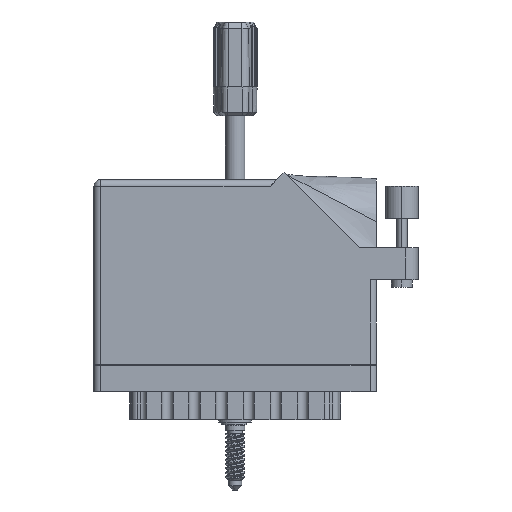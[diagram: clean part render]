
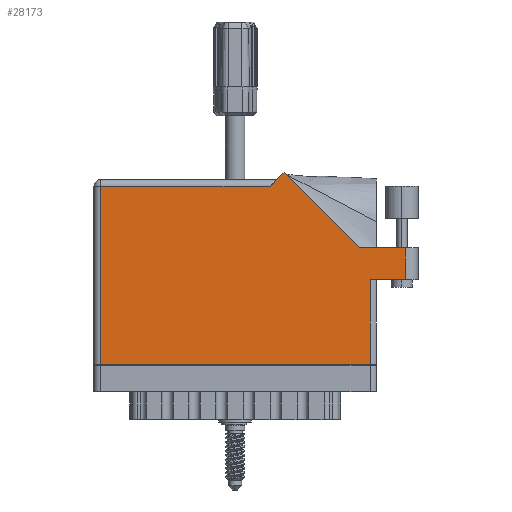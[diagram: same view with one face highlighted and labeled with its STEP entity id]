
A CAD part, front view. The second image highlights one B-rep face of the part: STEP entity #28173.
In plain terms, the highlighted face is planar.
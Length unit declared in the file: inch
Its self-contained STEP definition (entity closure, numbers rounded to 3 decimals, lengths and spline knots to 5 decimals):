
#412 = CARTESIAN_POINT ( 'NONE',  ( 2.656, 0.815, 0. ) ) ;
#1124 = EDGE_CURVE ( 'NONE', #15765, #76945, #48175, .T. ) ;
#2623 = VERTEX_POINT ( 'NONE', #39803 ) ;
#5084 = VECTOR ( 'NONE', #54343, 39.37008 ) ;
#5719 = DIRECTION ( 'NONE',  ( -0.707, 0.707, 0. ) ) ;
#6940 = VERTEX_POINT ( 'NONE', #26296 ) ;
#9632 = CARTESIAN_POINT ( 'NONE',  ( 0.062, 1.713, 0. ) ) ;
#9735 = CARTESIAN_POINT ( 'NONE',  ( 0.062, 0., 0. ) ) ;
#13336 = ORIENTED_EDGE ( 'NONE', *, *, #73205, .T. ) ;
#15765 = VERTEX_POINT ( 'NONE', #9632 ) ;
#18040 = EDGE_CURVE ( 'NONE', #20222, #15765, #36241, .T. ) ;
#18050 = CARTESIAN_POINT ( 'NONE',  ( 0.062, 0., 0. ) ) ;
#19052 = LINE ( 'NONE', #38894, #83810 ) ;
#19769 = EDGE_CURVE ( 'NONE', #76945, #59300, #78440, .T. ) ;
#19936 = LINE ( 'NONE', #37980, #72600 ) ;
#20222 = VERTEX_POINT ( 'NONE', #33118 ) ;
#21274 = ORIENTED_EDGE ( 'NONE', *, *, #50983, .T. ) ;
#21531 = CARTESIAN_POINT ( 'NONE',  ( 1.758, 1.775, 0. ) ) ;
#21573 = CARTESIAN_POINT ( 'NONE',  ( 3.118, 1.122, 0. ) ) ;
#22625 = DIRECTION ( 'NONE',  ( -0.707, -0.707, 0. ) ) ;
#22791 = LINE ( 'NONE', #21531, #33914 ) ;
#23823 = AXIS2_PLACEMENT_3D ( 'NONE', #49961, #63830, #77102 ) ;
#26296 = CARTESIAN_POINT ( 'NONE',  ( 1.82871, 1.84571, 0. ) ) ;
#26604 = DIRECTION ( 'NONE',  ( 0., 1., 0. ) ) ;
#27066 = ORIENTED_EDGE ( 'NONE', *, *, #1124, .T. ) ;
#28173 = ADVANCED_FACE ( 'NONE', ( #69219 ), #44003, .F. ) ;
#28233 = VERTEX_POINT ( 'NONE', #412 ) ;
#28353 = DIRECTION ( 'NONE',  ( 1., 0., 0. ) ) ;
#29772 = VECTOR ( 'NONE', #26604, 39.37008 ) ;
#31802 = LINE ( 'NONE', #52348, #29772 ) ;
#33118 = CARTESIAN_POINT ( 'NONE',  ( 1.696, 1.713, 0. ) ) ;
#33914 = VECTOR ( 'NONE', #22625, 39.37008 ) ;
#34187 = VECTOR ( 'NONE', #65042, 39.37008 ) ;
#34848 = VERTEX_POINT ( 'NONE', #76291 ) ;
#36241 = LINE ( 'NONE', #78296, #34187 ) ;
#37980 = CARTESIAN_POINT ( 'NONE',  ( 2.55242, 1.122, 0. ) ) ;
#38894 = CARTESIAN_POINT ( 'NONE',  ( 2.993, 1.122, 0. ) ) ;
#38897 = VECTOR ( 'NONE', #28353, 39.37008 ) ;
#39669 = ORIENTED_EDGE ( 'NONE', *, *, #68614, .T. ) ;
#39803 = CARTESIAN_POINT ( 'NONE',  ( 2.993, 0.815, 0. ) ) ;
#40502 = EDGE_CURVE ( 'NONE', #34848, #49420, #43546, .T. ) ;
#41000 = CARTESIAN_POINT ( 'NONE',  ( 2.718, 0.815, 0. ) ) ;
#41130 = LINE ( 'NONE', #41000, #70450 ) ;
#41555 = DIRECTION ( 'NONE',  ( 1., 0., 0. ) ) ;
#42440 = EDGE_CURVE ( 'NONE', #28233, #2623, #41130, .T. ) ;
#43546 = LINE ( 'NONE', #21573, #5084 ) ;
#44003 = PLANE ( 'NONE',  #23823 ) ;
#48175 = LINE ( 'NONE', #9735, #54243 ) ;
#49420 = VERTEX_POINT ( 'NONE', #59314 ) ;
#49961 = CARTESIAN_POINT ( 'NONE',  ( 0., 1.775, 0. ) ) ;
#50983 = EDGE_CURVE ( 'NONE', #2623, #34848, #19052, .T. ) ;
#51083 = EDGE_CURVE ( 'NONE', #49420, #6940, #19936, .T. ) ;
#52348 = CARTESIAN_POINT ( 'NONE',  ( 2.656, 0.815, 0. ) ) ;
#54243 = VECTOR ( 'NONE', #61533, 39.37008 ) ;
#54343 = DIRECTION ( 'NONE',  ( -1., 0., 0. ) ) ;
#54405 = ORIENTED_EDGE ( 'NONE', *, *, #19769, .T. ) ;
#57419 = ORIENTED_EDGE ( 'NONE', *, *, #51083, .T. ) ;
#59300 = VERTEX_POINT ( 'NONE', #83723 ) ;
#59314 = CARTESIAN_POINT ( 'NONE',  ( 2.55242, 1.122, 0. ) ) ;
#61533 = DIRECTION ( 'NONE',  ( 0., -1., 0. ) ) ;
#63830 = DIRECTION ( 'NONE',  ( 0., 0., -1. ) ) ;
#65042 = DIRECTION ( 'NONE',  ( -1., 0., 0. ) ) ;
#68614 = EDGE_CURVE ( 'NONE', #59300, #28233, #31802, .T. ) ;
#69037 = ORIENTED_EDGE ( 'NONE', *, *, #40502, .T. ) ;
#69219 = FACE_OUTER_BOUND ( 'NONE', #70929, .T. ) ;
#70245 = ORIENTED_EDGE ( 'NONE', *, *, #42440, .T. ) ;
#70450 = VECTOR ( 'NONE', #41555, 39.37008 ) ;
#70929 = EDGE_LOOP ( 'NONE', ( #70245, #21274, #69037, #57419, #13336, #72207, #27066, #54405, #39669 ) ) ;
#71446 = DIRECTION ( 'NONE',  ( 0., 1., 0. ) ) ;
#72207 = ORIENTED_EDGE ( 'NONE', *, *, #18040, .T. ) ;
#72600 = VECTOR ( 'NONE', #5719, 39.37008 ) ;
#73205 = EDGE_CURVE ( 'NONE', #6940, #20222, #22791, .T. ) ;
#73632 = CARTESIAN_POINT ( 'NONE',  ( 0., 0., 0. ) ) ;
#76291 = CARTESIAN_POINT ( 'NONE',  ( 2.993, 1.122, 0. ) ) ;
#76945 = VERTEX_POINT ( 'NONE', #18050 ) ;
#77102 = DIRECTION ( 'NONE',  ( -1., 0., 0. ) ) ;
#78296 = CARTESIAN_POINT ( 'NONE',  ( 0., 1.713, 0. ) ) ;
#78440 = LINE ( 'NONE', #73632, #38897 ) ;
#83723 = CARTESIAN_POINT ( 'NONE',  ( 2.656, 0., 0. ) ) ;
#83810 = VECTOR ( 'NONE', #71446, 39.37008 ) ;
